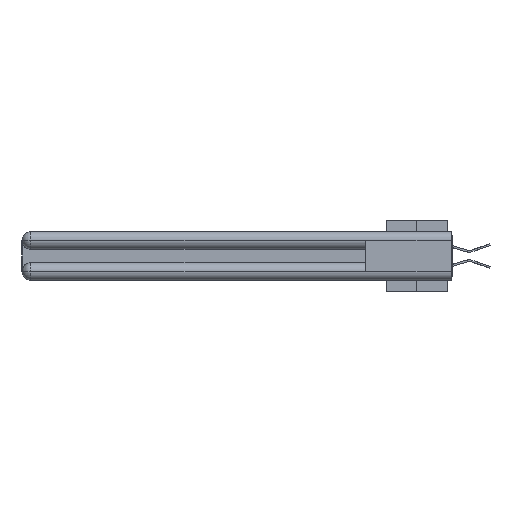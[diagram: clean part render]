
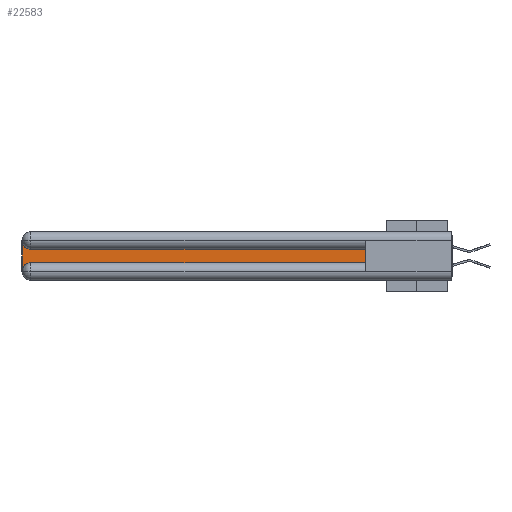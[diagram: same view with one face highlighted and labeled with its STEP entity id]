
A CAD part, left-side view. The second image highlights one B-rep face of the part: STEP entity #22583.
In plain terms, the highlighted planar face has unit normal (-1, 0, 0).
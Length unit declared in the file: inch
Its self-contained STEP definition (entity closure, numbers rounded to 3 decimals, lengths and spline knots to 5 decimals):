
#333 = ORIENTED_EDGE ( 'NONE', *, *, #30625, .T. ) ;
#2780 = CARTESIAN_POINT ( 'NONE',  ( 0.075, 0.6, -0.1225 ) ) ;
#3562 = AXIS2_PLACEMENT_3D ( 'NONE', #33213, #36317, #16035 ) ;
#5239 = ORIENTED_EDGE ( 'NONE', *, *, #18918, .T. ) ;
#5248 = CARTESIAN_POINT ( 'NONE',  ( 0.075, 2.94, -0.0625 ) ) ;
#5803 = CARTESIAN_POINT ( 'NONE',  ( 0.075, 3., -0.2175 ) ) ;
#6070 = ORIENTED_EDGE ( 'NONE', *, *, #31944, .T. ) ;
#9206 = ORIENTED_EDGE ( 'NONE', *, *, #26843, .T. ) ;
#9383 = VERTEX_POINT ( 'NONE', #9760 ) ;
#9668 = LINE ( 'NONE', #35648, #23440 ) ;
#9760 = CARTESIAN_POINT ( 'NONE',  ( 0.075, 0.6, -0.1225 ) ) ;
#10232 = AXIS2_PLACEMENT_3D ( 'NONE', #25959, #36055, #43168 ) ;
#12560 = VERTEX_POINT ( 'NONE', #20225 ) ;
#12630 = PLANE ( 'NONE',  #3562 ) ;
#13044 = VECTOR ( 'NONE', #26230, 39.37008 ) ;
#14103 = EDGE_CURVE ( 'NONE', #27197, #43197, #33755, .T. ) ;
#14764 = CARTESIAN_POINT ( 'NONE',  ( 0.075, 3., -0.0625 ) ) ;
#15520 = DIRECTION ( 'NONE',  ( 0., 0., -1. ) ) ;
#16035 = DIRECTION ( 'NONE',  ( 0., 0., -1. ) ) ;
#16042 = CARTESIAN_POINT ( 'NONE',  ( 0.075, 0.6, -0.2175 ) ) ;
#17544 = AXIS2_PLACEMENT_3D ( 'NONE', #5248, #29000, #15520 ) ;
#18313 = CIRCLE ( 'NONE', #10232, 0.06 ) ;
#18918 = EDGE_CURVE ( 'NONE', #12560, #9383, #41668, .T. ) ;
#19412 = LINE ( 'NONE', #5803, #13044 ) ;
#20225 = CARTESIAN_POINT ( 'NONE',  ( 0.075, 0.6, -0.2175 ) ) ;
#21838 = CARTESIAN_POINT ( 'NONE',  ( 0.075, 2.94, -0.1225 ) ) ;
#21855 = EDGE_CURVE ( 'NONE', #41962, #12560, #9668, .T. ) ;
#22583 = ADVANCED_FACE ( 'NONE', ( #36605 ), #12630, .F. ) ;
#22742 = ORIENTED_EDGE ( 'NONE', *, *, #14103, .T. ) ;
#23440 = VECTOR ( 'NONE', #25553, 39.37008 ) ;
#25553 = DIRECTION ( 'NONE',  ( 0., -1., 0. ) ) ;
#25847 = VERTEX_POINT ( 'NONE', #26188 ) ;
#25959 = CARTESIAN_POINT ( 'NONE',  ( 0.075, 2.94, -0.2775 ) ) ;
#26188 = CARTESIAN_POINT ( 'NONE',  ( 0.075, 3., -0.2775 ) ) ;
#26230 = DIRECTION ( 'NONE',  ( 0., 0., -1. ) ) ;
#26843 = EDGE_CURVE ( 'NONE', #43197, #25847, #19412, .T. ) ;
#27197 = VERTEX_POINT ( 'NONE', #21838 ) ;
#27202 = LINE ( 'NONE', #2780, #32523 ) ;
#29000 = DIRECTION ( 'NONE',  ( 1., 0., 0. ) ) ;
#29372 = DIRECTION ( 'NONE',  ( 0., 1., 0. ) ) ;
#30625 = EDGE_CURVE ( 'NONE', #25847, #41962, #18313, .T. ) ;
#31944 = EDGE_CURVE ( 'NONE', #9383, #27197, #27202, .T. ) ;
#32523 = VECTOR ( 'NONE', #29372, 39.37008 ) ;
#32825 = ORIENTED_EDGE ( 'NONE', *, *, #21855, .T. ) ;
#32864 = CARTESIAN_POINT ( 'NONE',  ( 0.075, 2.94, -0.2175 ) ) ;
#33213 = CARTESIAN_POINT ( 'NONE',  ( 0.075, 3., -0.1225 ) ) ;
#33755 = CIRCLE ( 'NONE', #17544, 0.06 ) ;
#35648 = CARTESIAN_POINT ( 'NONE',  ( 0.075, 0.6, -0.2175 ) ) ;
#36055 = DIRECTION ( 'NONE',  ( 1., 0., 0. ) ) ;
#36317 = DIRECTION ( 'NONE',  ( 1., 0., 0. ) ) ;
#36605 = FACE_OUTER_BOUND ( 'NONE', #42760, .T. ) ;
#39019 = VECTOR ( 'NONE', #43140, 39.37008 ) ;
#41668 = LINE ( 'NONE', #16042, #39019 ) ;
#41962 = VERTEX_POINT ( 'NONE', #32864 ) ;
#42760 = EDGE_LOOP ( 'NONE', ( #6070, #22742, #9206, #333, #32825, #5239 ) ) ;
#43140 = DIRECTION ( 'NONE',  ( 0., 0., 1. ) ) ;
#43168 = DIRECTION ( 'NONE',  ( 0., 0., -1. ) ) ;
#43197 = VERTEX_POINT ( 'NONE', #14764 ) ;
